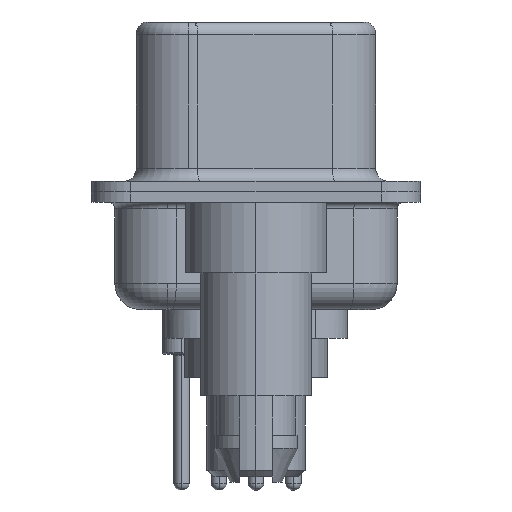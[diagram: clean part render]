
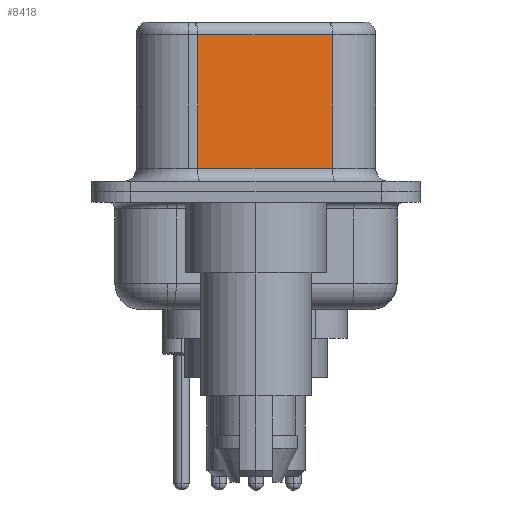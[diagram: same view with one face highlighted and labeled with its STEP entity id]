
A CAD part, left-side view. The second image highlights one B-rep face of the part: STEP entity #8418.
In plain terms, the highlighted planar face has unit normal (-0.985, -0.174, 0).
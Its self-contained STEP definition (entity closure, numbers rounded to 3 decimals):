
#409 = VERTEX_POINT ( 'NONE', #16882 ) ;
#1353 = VERTEX_POINT ( 'NONE', #19903 ) ;
#3093 = VECTOR ( 'NONE', #24467, 1000. ) ;
#4486 = DIRECTION ( 'NONE',  ( 0.174, -0.985, 0. ) ) ;
#4793 = ORIENTED_EDGE ( 'NONE', *, *, #13477, .T. ) ;
#5775 = VECTOR ( 'NONE', #9991, 1000. ) ;
#6110 = VECTOR ( 'NONE', #4486, 1000. ) ;
#6938 = CARTESIAN_POINT ( 'NONE',  ( 4.58, -2.927, 6.02 ) ) ;
#8165 = CARTESIAN_POINT ( 'NONE',  ( 3.67, 2.233, 6.52 ) ) ;
#8382 = VECTOR ( 'NONE', #23760, 1000. ) ;
#8418 = ADVANCED_FACE ( 'NONE', ( #18772 ), #24507, .F. ) ;
#8874 = CARTESIAN_POINT ( 'NONE',  ( 4.58, -2.927, 6.52 ) ) ;
#8939 = LINE ( 'NONE', #8874, #3093 ) ;
#9991 = DIRECTION ( 'NONE',  ( -0.174, 0.985, 0. ) ) ;
#10933 = LINE ( 'NONE', #23662, #5775 ) ;
#13362 = DIRECTION ( 'NONE',  ( -0.174, 0.985, 0. ) ) ;
#13419 = DIRECTION ( 'NONE',  ( 0.985, 0.174, 0. ) ) ;
#13477 = EDGE_CURVE ( 'NONE', #23189, #14275, #10933, .T. ) ;
#13550 = CARTESIAN_POINT ( 'NONE',  ( 4.58, -2.927, 6.52 ) ) ;
#13731 = EDGE_LOOP ( 'NONE', ( #16988, #4793, #18616, #20698 ) ) ;
#14163 = CARTESIAN_POINT ( 'NONE',  ( 4.58, -2.927, 0.9 ) ) ;
#14275 = VERTEX_POINT ( 'NONE', #21952 ) ;
#16481 = LINE ( 'NONE', #14163, #6110 ) ;
#16882 = CARTESIAN_POINT ( 'NONE',  ( 3.67, 2.233, 0.9 ) ) ;
#16988 = ORIENTED_EDGE ( 'NONE', *, *, #24992, .F. ) ;
#17147 = EDGE_CURVE ( 'NONE', #409, #1353, #16481, .T. ) ;
#18616 = ORIENTED_EDGE ( 'NONE', *, *, #22860, .T. ) ;
#18772 = FACE_OUTER_BOUND ( 'NONE', #13731, .T. ) ;
#19903 = CARTESIAN_POINT ( 'NONE',  ( 4.58, -2.927, 0.9 ) ) ;
#20698 = ORIENTED_EDGE ( 'NONE', *, *, #17147, .T. ) ;
#21952 = CARTESIAN_POINT ( 'NONE',  ( 3.67, 2.233, 6.02 ) ) ;
#22860 = EDGE_CURVE ( 'NONE', #14275, #409, #23336, .T. ) ;
#23187 = AXIS2_PLACEMENT_3D ( 'NONE', #13550, #13419, #13362 ) ;
#23189 = VERTEX_POINT ( 'NONE', #6938 ) ;
#23336 = LINE ( 'NONE', #8165, #8382 ) ;
#23662 = CARTESIAN_POINT ( 'NONE',  ( 4.58, -2.927, 6.02 ) ) ;
#23760 = DIRECTION ( 'NONE',  ( 0., 0., -1. ) ) ;
#24467 = DIRECTION ( 'NONE',  ( 0., 0., -1. ) ) ;
#24507 = PLANE ( 'NONE',  #23187 ) ;
#24992 = EDGE_CURVE ( 'NONE', #23189, #1353, #8939, .T. ) ;
